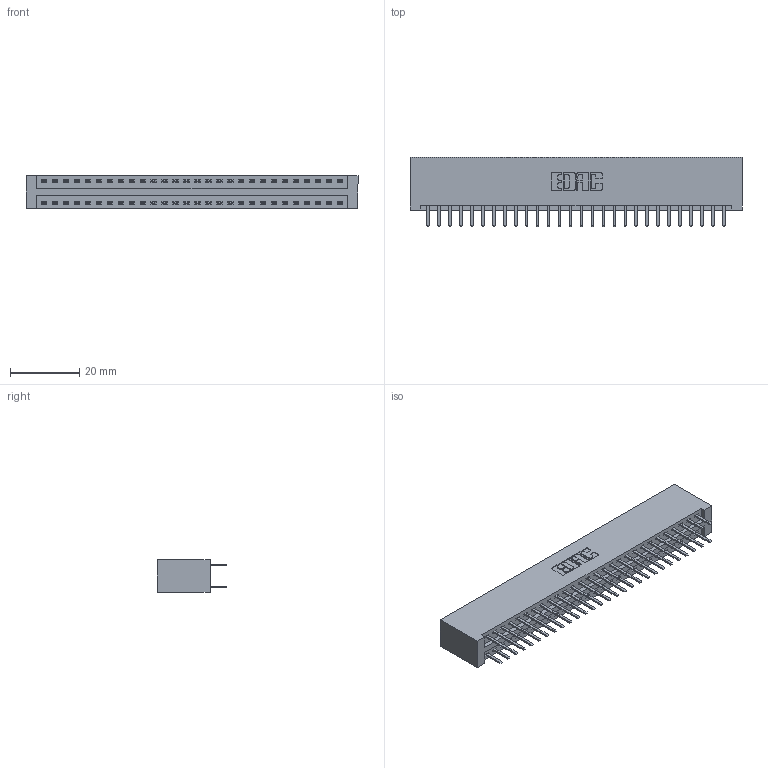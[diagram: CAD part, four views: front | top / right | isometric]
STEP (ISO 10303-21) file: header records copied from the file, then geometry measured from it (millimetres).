
FILE_DESCRIPTION (( 'STEP AP203' ), '1' );
FILE_NAME ('346-056-520-201.STEP', '2018-08-28T02:12:27', ( '' ), ( '' ), 'SwSTEP 2.0', 'SolidWorks 2016', '' );
FILE_SCHEMA (( 'CONFIG_CONTROL_DESIGN' ));
Length unit declared in the file: inch
Products named in the file (3): 346 Part_No Mounting Lugs; 345-292-001_345-293-120; 346-056-520-201
Assembly tree (57 placements, depth 2):
  346-056-520-201
    346 Part_No Mounting Lugs
    345-292-001_345-293-120  x56
Bounding box: 96.14 x 20.02 x 9.4 mm (x, y, z)
Volume: 9814.7 mm3; surface area: 13376.4 mm2
Topology: 57 solids, 57 shells, 3250 faces, 9433 edges, 6138 vertices
Faces by surface type: plane 2144, cylinder 1106
Entity records: 19995 total; most frequent: CARTESIAN_POINT 3324, ORIENTED_EDGE 3246, DIRECTION 2963, EDGE_CURVE 1623, VECTOR 1383, LINE 1383, VERTEX_POINT 1078, AXIS2_PLACEMENT_3D 790
